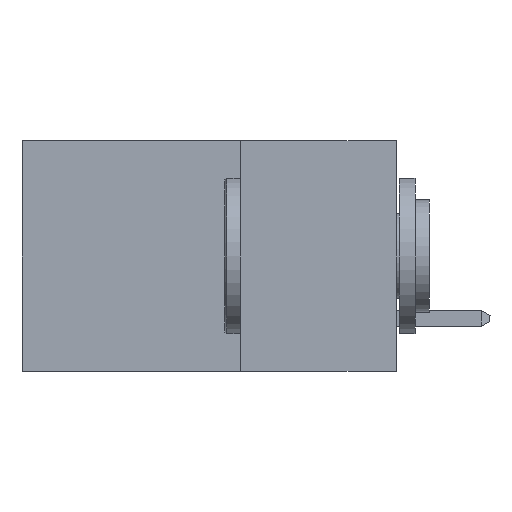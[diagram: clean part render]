
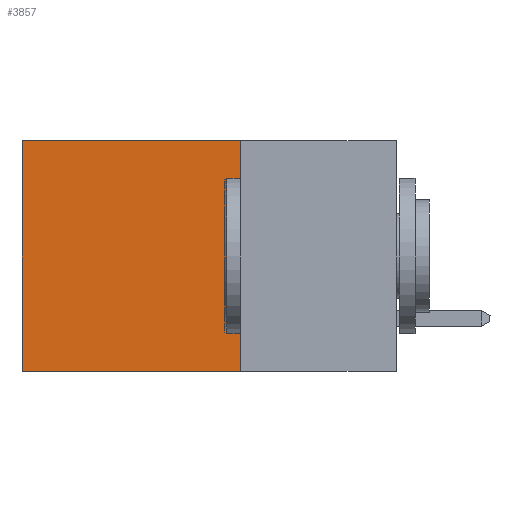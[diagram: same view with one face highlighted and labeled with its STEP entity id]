
A CAD part, left-side view. The second image highlights one B-rep face of the part: STEP entity #3857.
In plain terms, the highlighted planar face has unit normal (-1, 0, 0).
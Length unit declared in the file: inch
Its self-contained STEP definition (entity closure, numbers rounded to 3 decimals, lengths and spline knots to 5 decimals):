
#67 = CARTESIAN_POINT ( 'NONE',  ( 0.2615, 0.25, -0.37 ) ) ;
#1399 = CARTESIAN_POINT ( 'NONE',  ( 0.2615, 0.25, -0.37 ) ) ;
#2207 = CARTESIAN_POINT ( 'NONE',  ( 0.2615, 0.6, 0. ) ) ;
#2413 = VERTEX_POINT ( 'NONE', #2207 ) ;
#3419 = EDGE_CURVE ( 'NONE', #2413, #3936, #13286, .T. ) ;
#3558 = CARTESIAN_POINT ( 'NONE',  ( 0.2615, 0.25, 0. ) ) ;
#3568 = CARTESIAN_POINT ( 'NONE',  ( 0.2615, 0.25, 0. ) ) ;
#3651 = LINE ( 'NONE', #10885, #13242 ) ;
#3670 = ORIENTED_EDGE ( 'NONE', *, *, #9180, .T. ) ;
#3832 = EDGE_CURVE ( 'NONE', #10908, #12968, #3651, .T. ) ;
#3857 = ADVANCED_FACE ( 'NONE', ( #8263 ), #5085, .F. ) ;
#3936 = VERTEX_POINT ( 'NONE', #11145 ) ;
#4204 = DIRECTION ( 'NONE',  ( 0., 0., -1. ) ) ;
#4581 = LINE ( 'NONE', #3568, #5665 ) ;
#4739 = DIRECTION ( 'NONE',  ( 0., 0., -1. ) ) ;
#5085 = PLANE ( 'NONE',  #11526 ) ;
#5230 = VECTOR ( 'NONE', #5509, 39.37008 ) ;
#5509 = DIRECTION ( 'NONE',  ( 0., 1., 0. ) ) ;
#5665 = VECTOR ( 'NONE', #8708, 39.37008 ) ;
#6521 = ORIENTED_EDGE ( 'NONE', *, *, #12193, .F. ) ;
#6563 = ORIENTED_EDGE ( 'NONE', *, *, #3832, .F. ) ;
#7751 = ORIENTED_EDGE ( 'NONE', *, *, #3419, .T. ) ;
#8263 = FACE_OUTER_BOUND ( 'NONE', #9404, .T. ) ;
#8708 = DIRECTION ( 'NONE',  ( 0., 1., 0. ) ) ;
#9132 = DIRECTION ( 'NONE',  ( 1., 0., 0. ) ) ;
#9180 = EDGE_CURVE ( 'NONE', #10908, #2413, #4581, .T. ) ;
#9404 = EDGE_LOOP ( 'NONE', ( #7751, #6521, #6563, #3670 ) ) ;
#10650 = LINE ( 'NONE', #1399, #5230 ) ;
#10885 = CARTESIAN_POINT ( 'NONE',  ( 0.2615, 0.25, -0.37 ) ) ;
#10908 = VERTEX_POINT ( 'NONE', #3558 ) ;
#11128 = CARTESIAN_POINT ( 'NONE',  ( 0.2615, 0.6, -0.37 ) ) ;
#11145 = CARTESIAN_POINT ( 'NONE',  ( 0.2615, 0.6, -0.37 ) ) ;
#11526 = AXIS2_PLACEMENT_3D ( 'NONE', #67, #9132, #4204 ) ;
#11940 = VECTOR ( 'NONE', #12282, 39.37008 ) ;
#12193 = EDGE_CURVE ( 'NONE', #12968, #3936, #10650, .T. ) ;
#12282 = DIRECTION ( 'NONE',  ( 0., 0., -1. ) ) ;
#12813 = CARTESIAN_POINT ( 'NONE',  ( 0.2615, 0.25, -0.37 ) ) ;
#12968 = VERTEX_POINT ( 'NONE', #12813 ) ;
#13242 = VECTOR ( 'NONE', #4739, 39.37008 ) ;
#13286 = LINE ( 'NONE', #11128, #11940 ) ;
